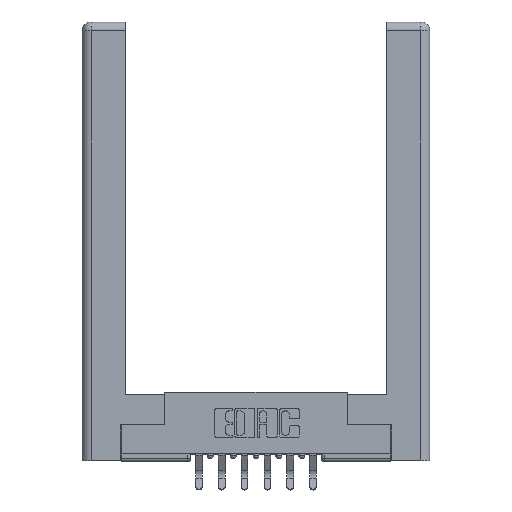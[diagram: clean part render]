
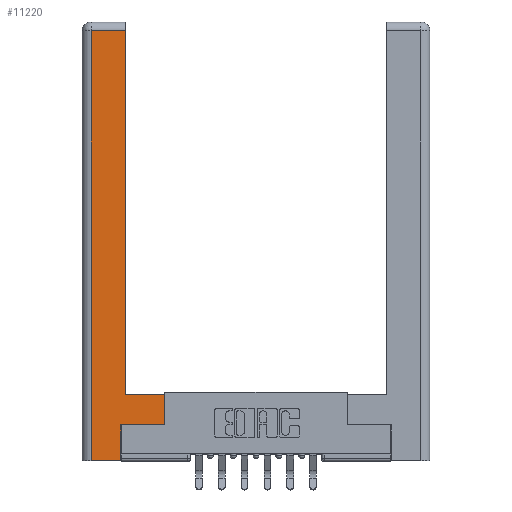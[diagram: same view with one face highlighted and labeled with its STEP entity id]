
A CAD part, top view. The second image highlights one B-rep face of the part: STEP entity #11220.
In plain terms, the highlighted planar face has unit normal (0, 0, 1).
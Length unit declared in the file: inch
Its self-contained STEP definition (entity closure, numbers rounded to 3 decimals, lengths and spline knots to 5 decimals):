
#129 = DIRECTION ( 'NONE',  ( 1., 0., 0. ) ) ;
#187 = EDGE_CURVE ( 'NONE', #4279, #7406, #7806, .T. ) ;
#347 = ORIENTED_EDGE ( 'NONE', *, *, #11428, .T. ) ;
#396 = CARTESIAN_POINT ( 'NONE',  ( 0.0615, 2.94, 0. ) ) ;
#581 = ORIENTED_EDGE ( 'NONE', *, *, #11938, .T. ) ;
#764 = EDGE_LOOP ( 'NONE', ( #4996, #347, #5018, #10487, #7358, #11227, #581, #1130 ) ) ;
#1066 = LINE ( 'NONE', #5952, #9843 ) ;
#1130 = ORIENTED_EDGE ( 'NONE', *, *, #5666, .T. ) ;
#1735 = VECTOR ( 'NONE', #10043, 39.37008 ) ;
#2181 = LINE ( 'NONE', #10079, #1735 ) ;
#2809 = FACE_OUTER_BOUND ( 'NONE', #764, .T. ) ;
#3052 = DIRECTION ( 'NONE',  ( 0., 1., 0. ) ) ;
#3210 = CARTESIAN_POINT ( 'NONE',  ( 0., 0., 0. ) ) ;
#3749 = LINE ( 'NONE', #4713, #9208 ) ;
#3917 = EDGE_CURVE ( 'NONE', #8266, #4743, #10580, .T. ) ;
#4026 = CARTESIAN_POINT ( 'NONE',  ( 0.565, 0.245, 0. ) ) ;
#4054 = CARTESIAN_POINT ( 'NONE',  ( 0.265, 0.245, 0. ) ) ;
#4062 = VECTOR ( 'NONE', #129, 39.37008 ) ;
#4087 = VECTOR ( 'NONE', #8948, 39.37008 ) ;
#4103 = CARTESIAN_POINT ( 'NONE',  ( 0.295, 2.94, 0. ) ) ;
#4156 = DIRECTION ( 'NONE',  ( 0., 0., -1. ) ) ;
#4279 = VERTEX_POINT ( 'NONE', #5431 ) ;
#4401 = CARTESIAN_POINT ( 'NONE',  ( 0.0615, 0., 0. ) ) ;
#4445 = CARTESIAN_POINT ( 'NONE',  ( 0.0615, 2.94, 0. ) ) ;
#4685 = VERTEX_POINT ( 'NONE', #8082 ) ;
#4713 = CARTESIAN_POINT ( 'NONE',  ( 0.265, 0., 0. ) ) ;
#4743 = VERTEX_POINT ( 'NONE', #4401 ) ;
#4996 = ORIENTED_EDGE ( 'NONE', *, *, #8105, .T. ) ;
#5018 = ORIENTED_EDGE ( 'NONE', *, *, #3917, .T. ) ;
#5164 = DIRECTION ( 'NONE',  ( -1., 0., 0. ) ) ;
#5431 = CARTESIAN_POINT ( 'NONE',  ( 0.265, 0., 0. ) ) ;
#5596 = LINE ( 'NONE', #4026, #4062 ) ;
#5666 = EDGE_CURVE ( 'NONE', #4685, #12358, #2181, .T. ) ;
#5952 = CARTESIAN_POINT ( 'NONE',  ( 0.295, 3., 0. ) ) ;
#6526 = CARTESIAN_POINT ( 'NONE',  ( 0.295, 0.45, 0. ) ) ;
#6994 = AXIS2_PLACEMENT_3D ( 'NONE', #3210, #4156, #5164 ) ;
#7358 = ORIENTED_EDGE ( 'NONE', *, *, #187, .T. ) ;
#7362 = VERTEX_POINT ( 'NONE', #4103 ) ;
#7406 = VERTEX_POINT ( 'NONE', #4054 ) ;
#7500 = VECTOR ( 'NONE', #7985, 39.37008 ) ;
#7522 = VECTOR ( 'NONE', #12184, 39.37008 ) ;
#7651 = DIRECTION ( 'NONE',  ( 1., 0., 0. ) ) ;
#7806 = LINE ( 'NONE', #11910, #7500 ) ;
#7985 = DIRECTION ( 'NONE',  ( 0., 1., 0. ) ) ;
#8082 = CARTESIAN_POINT ( 'NONE',  ( 0.565, 0.45, 0. ) ) ;
#8105 = EDGE_CURVE ( 'NONE', #12358, #7362, #1066, .T. ) ;
#8266 = VERTEX_POINT ( 'NONE', #396 ) ;
#8302 = CARTESIAN_POINT ( 'NONE',  ( 0.565, 0.245, 0. ) ) ;
#8720 = VECTOR ( 'NONE', #9730, 39.37008 ) ;
#8812 = CARTESIAN_POINT ( 'NONE',  ( 0.565, 0.45, 0. ) ) ;
#8948 = DIRECTION ( 'NONE',  ( 0., -1., 0. ) ) ;
#8985 = CARTESIAN_POINT ( 'NONE',  ( 0.0615, 0., 0. ) ) ;
#9208 = VECTOR ( 'NONE', #7651, 39.37008 ) ;
#9324 = EDGE_CURVE ( 'NONE', #7406, #9520, #5596, .T. ) ;
#9479 = LINE ( 'NONE', #4445, #7522 ) ;
#9520 = VERTEX_POINT ( 'NONE', #8302 ) ;
#9730 = DIRECTION ( 'NONE',  ( 0., 1., 0. ) ) ;
#9843 = VECTOR ( 'NONE', #3052, 39.37008 ) ;
#10043 = DIRECTION ( 'NONE',  ( -1., 0., 0. ) ) ;
#10079 = CARTESIAN_POINT ( 'NONE',  ( 0.295, 0.45, 0. ) ) ;
#10364 = EDGE_CURVE ( 'NONE', #4743, #4279, #3749, .T. ) ;
#10487 = ORIENTED_EDGE ( 'NONE', *, *, #10364, .T. ) ;
#10580 = LINE ( 'NONE', #8985, #4087 ) ;
#10914 = PLANE ( 'NONE',  #6994 ) ;
#11220 = ADVANCED_FACE ( 'NONE', ( #2809 ), #10914, .F. ) ;
#11227 = ORIENTED_EDGE ( 'NONE', *, *, #9324, .T. ) ;
#11281 = LINE ( 'NONE', #8812, #8720 ) ;
#11428 = EDGE_CURVE ( 'NONE', #7362, #8266, #9479, .T. ) ;
#11910 = CARTESIAN_POINT ( 'NONE',  ( 0.265, 0.245, 0. ) ) ;
#11938 = EDGE_CURVE ( 'NONE', #9520, #4685, #11281, .T. ) ;
#12184 = DIRECTION ( 'NONE',  ( -1., 0., 0. ) ) ;
#12358 = VERTEX_POINT ( 'NONE', #6526 ) ;
